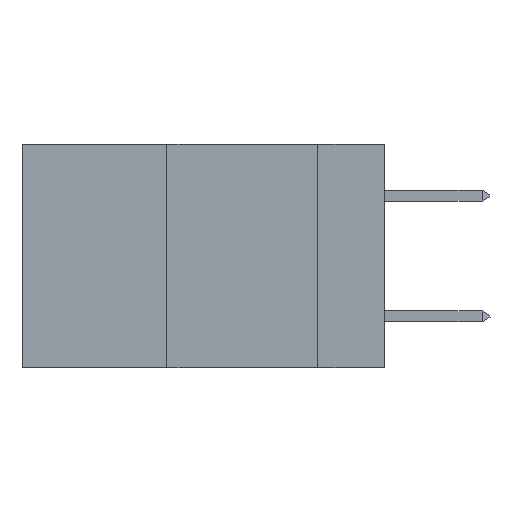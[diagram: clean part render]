
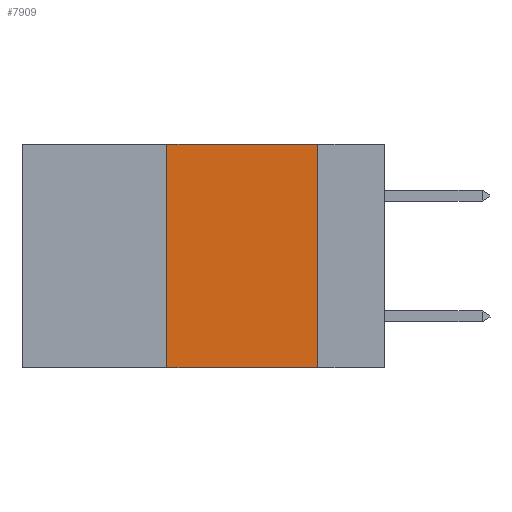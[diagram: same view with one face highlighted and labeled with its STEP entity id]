
A CAD part, left-side view. The second image highlights one B-rep face of the part: STEP entity #7909.
In plain terms, the highlighted planar face has unit normal (-1, 0, 0).
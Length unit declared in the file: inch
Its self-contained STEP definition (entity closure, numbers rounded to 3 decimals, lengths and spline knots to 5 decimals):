
#395 = AXIS2_PLACEMENT_3D ( 'NONE', #14692, #16172, #7176 ) ;
#550 = VERTEX_POINT ( 'NONE', #10266 ) ;
#1541 = VERTEX_POINT ( 'NONE', #17283 ) ;
#3325 = CARTESIAN_POINT ( 'NONE',  ( 0., 0.11, -0.37 ) ) ;
#3922 = EDGE_LOOP ( 'NONE', ( #8083, #16989, #5495, #18378 ) ) ;
#3938 = VERTEX_POINT ( 'NONE', #18749 ) ;
#4220 = CARTESIAN_POINT ( 'NONE',  ( 0., 0.36, 0. ) ) ;
#4582 = DIRECTION ( 'NONE',  ( 0., 0., -1. ) ) ;
#5029 = EDGE_CURVE ( 'NONE', #550, #11607, #12211, .T. ) ;
#5495 = ORIENTED_EDGE ( 'NONE', *, *, #13442, .F. ) ;
#6601 = DIRECTION ( 'NONE',  ( 0., -1., 0. ) ) ;
#7176 = DIRECTION ( 'NONE',  ( 0., 0., -1. ) ) ;
#7197 = VECTOR ( 'NONE', #4582, 39.37008 ) ;
#7909 = ADVANCED_FACE ( 'NONE', ( #12548 ), #13166, .F. ) ;
#8083 = ORIENTED_EDGE ( 'NONE', *, *, #12454, .F. ) ;
#8202 = VECTOR ( 'NONE', #15564, 39.37008 ) ;
#9814 = EDGE_CURVE ( 'NONE', #1541, #3938, #11037, .T. ) ;
#10266 = CARTESIAN_POINT ( 'NONE',  ( 0., 0.36, -0.37 ) ) ;
#10572 = VECTOR ( 'NONE', #6601, 39.37008 ) ;
#10917 = LINE ( 'NONE', #4220, #18829 ) ;
#11037 = LINE ( 'NONE', #12593, #10572 ) ;
#11607 = VERTEX_POINT ( 'NONE', #3325 ) ;
#12211 = LINE ( 'NONE', #18472, #8202 ) ;
#12454 = EDGE_CURVE ( 'NONE', #3938, #11607, #19102, .T. ) ;
#12548 = FACE_OUTER_BOUND ( 'NONE', #3922, .T. ) ;
#12593 = CARTESIAN_POINT ( 'NONE',  ( 0., 0.6, 0. ) ) ;
#13166 = PLANE ( 'NONE',  #395 ) ;
#13442 = EDGE_CURVE ( 'NONE', #550, #1541, #10917, .T. ) ;
#13553 = CARTESIAN_POINT ( 'NONE',  ( 0., 0.11, 0. ) ) ;
#14692 = CARTESIAN_POINT ( 'NONE',  ( 0., 0.6, 0. ) ) ;
#14724 = DIRECTION ( 'NONE',  ( 0., 0., 1. ) ) ;
#15564 = DIRECTION ( 'NONE',  ( 0., -1., 0. ) ) ;
#16172 = DIRECTION ( 'NONE',  ( 1., 0., 0. ) ) ;
#16989 = ORIENTED_EDGE ( 'NONE', *, *, #9814, .F. ) ;
#17283 = CARTESIAN_POINT ( 'NONE',  ( 0., 0.36, 0. ) ) ;
#18378 = ORIENTED_EDGE ( 'NONE', *, *, #5029, .T. ) ;
#18472 = CARTESIAN_POINT ( 'NONE',  ( 0., 0.6, -0.37 ) ) ;
#18749 = CARTESIAN_POINT ( 'NONE',  ( 0., 0.11, 0. ) ) ;
#18829 = VECTOR ( 'NONE', #14724, 39.37008 ) ;
#19102 = LINE ( 'NONE', #13553, #7197 ) ;
